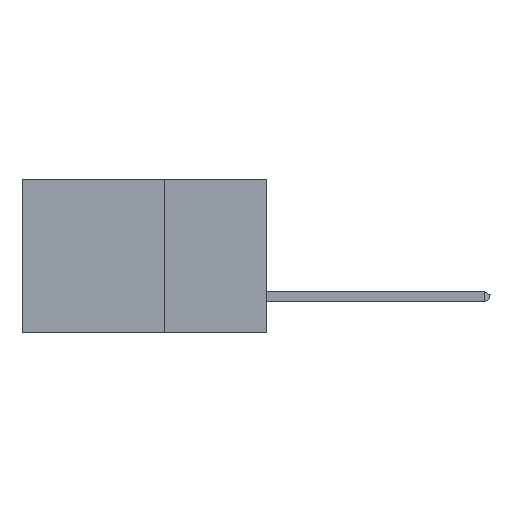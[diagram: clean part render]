
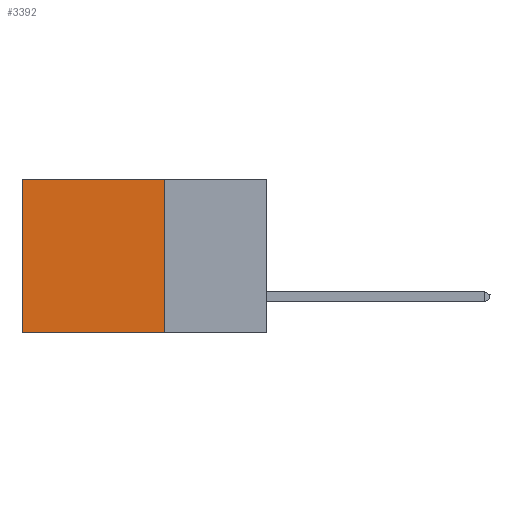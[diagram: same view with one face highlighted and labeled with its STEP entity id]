
A CAD part, left-side view. The second image highlights one B-rep face of the part: STEP entity #3392.
In plain terms, the highlighted planar face has unit normal (-1, 0, 0).
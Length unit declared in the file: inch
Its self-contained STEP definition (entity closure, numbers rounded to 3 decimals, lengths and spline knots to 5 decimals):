
#439 = ORIENTED_EDGE ( 'NONE', *, *, #1105, .F. ) ;
#443 = DIRECTION ( 'NONE',  ( 0., 0., -1. ) ) ;
#1034 = EDGE_CURVE ( 'NONE', #6201, #3914, #6302, .T. ) ;
#1055 = DIRECTION ( 'NONE',  ( 0., 1., 0. ) ) ;
#1105 = EDGE_CURVE ( 'NONE', #3914, #3742, #4909, .T. ) ;
#1172 = VECTOR ( 'NONE', #1055, 39.37008 ) ;
#1973 = CARTESIAN_POINT ( 'NONE',  ( 0.2875, 0.25, -0.375 ) ) ;
#2054 = CARTESIAN_POINT ( 'NONE',  ( 0.2875, 0.6, -0.375 ) ) ;
#2421 = VERTEX_POINT ( 'NONE', #4675 ) ;
#2625 = CARTESIAN_POINT ( 'NONE',  ( 0.2875, 0.25, 0. ) ) ;
#2924 = ORIENTED_EDGE ( 'NONE', *, *, #1034, .F. ) ;
#3339 = EDGE_LOOP ( 'NONE', ( #3679, #439, #2924, #9159 ) ) ;
#3392 = ADVANCED_FACE ( 'NONE', ( #7192 ), #6590, .F. ) ;
#3525 = LINE ( 'NONE', #9313, #8462 ) ;
#3529 = VECTOR ( 'NONE', #7142, 39.37008 ) ;
#3620 = EDGE_CURVE ( 'NONE', #6201, #2421, #5093, .T. ) ;
#3679 = ORIENTED_EDGE ( 'NONE', *, *, #6189, .T. ) ;
#3742 = VERTEX_POINT ( 'NONE', #2054 ) ;
#3767 = DIRECTION ( 'NONE',  ( 0., 0., -1. ) ) ;
#3914 = VERTEX_POINT ( 'NONE', #8889 ) ;
#3994 = VECTOR ( 'NONE', #7178, 39.37008 ) ;
#4675 = CARTESIAN_POINT ( 'NONE',  ( 0.2875, 0.6, 0. ) ) ;
#4751 = CARTESIAN_POINT ( 'NONE',  ( 0.2875, 0.25, 0. ) ) ;
#4801 = AXIS2_PLACEMENT_3D ( 'NONE', #7313, #8805, #3767 ) ;
#4909 = LINE ( 'NONE', #7769, #3994 ) ;
#5093 = LINE ( 'NONE', #4751, #1172 ) ;
#6189 = EDGE_CURVE ( 'NONE', #2421, #3742, #3525, .T. ) ;
#6201 = VERTEX_POINT ( 'NONE', #2625 ) ;
#6302 = LINE ( 'NONE', #1973, #3529 ) ;
#6590 = PLANE ( 'NONE',  #4801 ) ;
#7142 = DIRECTION ( 'NONE',  ( 0., 0., -1. ) ) ;
#7178 = DIRECTION ( 'NONE',  ( 0., 1., 0. ) ) ;
#7192 = FACE_OUTER_BOUND ( 'NONE', #3339, .T. ) ;
#7313 = CARTESIAN_POINT ( 'NONE',  ( 0.2875, 0.25, -0.375 ) ) ;
#7769 = CARTESIAN_POINT ( 'NONE',  ( 0.2875, 0.25, -0.375 ) ) ;
#8462 = VECTOR ( 'NONE', #443, 39.37008 ) ;
#8805 = DIRECTION ( 'NONE',  ( 1., 0., 0. ) ) ;
#8889 = CARTESIAN_POINT ( 'NONE',  ( 0.2875, 0.25, -0.375 ) ) ;
#9159 = ORIENTED_EDGE ( 'NONE', *, *, #3620, .T. ) ;
#9313 = CARTESIAN_POINT ( 'NONE',  ( 0.2875, 0.6, -0.375 ) ) ;
